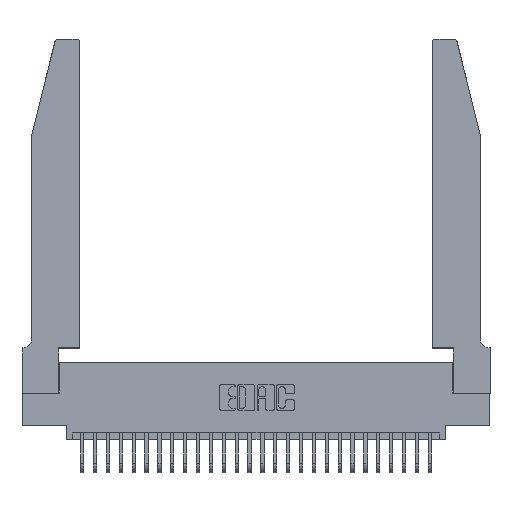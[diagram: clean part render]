
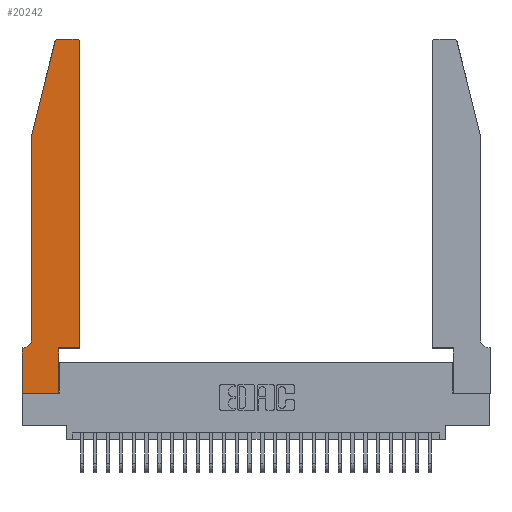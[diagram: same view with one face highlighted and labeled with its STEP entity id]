
A CAD part, top view. The second image highlights one B-rep face of the part: STEP entity #20242.
In plain terms, the highlighted planar face has unit normal (0, 0, 1).
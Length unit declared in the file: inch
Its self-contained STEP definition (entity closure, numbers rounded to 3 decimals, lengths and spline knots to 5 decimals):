
#351 = CARTESIAN_POINT ( 'NONE',  ( 0.2605, 2.75, 0.37 ) ) ;
#544 = DIRECTION ( 'NONE',  ( -1., 0., 0. ) ) ;
#545 = FACE_OUTER_BOUND ( 'NONE', #12466, .T. ) ;
#628 = VECTOR ( 'NONE', #4740, 39.37008 ) ;
#703 = VERTEX_POINT ( 'NONE', #11241 ) ;
#746 = VERTEX_POINT ( 'NONE', #26456 ) ;
#1192 = AXIS2_PLACEMENT_3D ( 'NONE', #9117, #24202, #11315 ) ;
#1303 = CARTESIAN_POINT ( 'NONE',  ( 0.284, 2.75, 0.37 ) ) ;
#1396 = AXIS2_PLACEMENT_3D ( 'NONE', #6137, #21245, #8283 ) ;
#2359 = DIRECTION ( 'NONE',  ( 1., 0., 0. ) ) ;
#2407 = EDGE_CURVE ( 'NONE', #12061, #4541, #15665, .T. ) ;
#2784 = ORIENTED_EDGE ( 'NONE', *, *, #23718, .T. ) ;
#3391 = LINE ( 'NONE', #25448, #25352 ) ;
#3420 = VECTOR ( 'NONE', #4451, 39.37008 ) ;
#3762 = VERTEX_POINT ( 'NONE', #19898 ) ;
#4040 = VERTEX_POINT ( 'NONE', #1303 ) ;
#4061 = CARTESIAN_POINT ( 'NONE',  ( 0.4505, 0.35, 0.37 ) ) ;
#4200 = ORIENTED_EDGE ( 'NONE', *, *, #19794, .T. ) ;
#4275 = CARTESIAN_POINT ( 'NONE',  ( 0.4505, 2.72, 0.37 ) ) ;
#4295 = VERTEX_POINT ( 'NONE', #4275 ) ;
#4451 = DIRECTION ( 'NONE',  ( 0., -1., 0. ) ) ;
#4541 = VERTEX_POINT ( 'NONE', #7356 ) ;
#4579 = CARTESIAN_POINT ( 'NONE',  ( 0., 0., 0.37 ) ) ;
#4740 = DIRECTION ( 'NONE',  ( -1., 0., 0. ) ) ;
#5002 = DIRECTION ( 'NONE',  ( 0., -1., 0. ) ) ;
#5153 = EDGE_CURVE ( 'NONE', #18616, #25102, #11440, .T. ) ;
#5205 = VECTOR ( 'NONE', #8239, 39.37008 ) ;
#5359 = VERTEX_POINT ( 'NONE', #17204 ) ;
#5669 = EDGE_CURVE ( 'NONE', #25165, #4295, #27196, .T. ) ;
#5719 = ORIENTED_EDGE ( 'NONE', *, *, #19094, .T. ) ;
#6094 = CARTESIAN_POINT ( 'NONE',  ( 0.2865, 0.35, 0.37 ) ) ;
#6135 = AXIS2_PLACEMENT_3D ( 'NONE', #13199, #8810, #2359 ) ;
#6137 = CARTESIAN_POINT ( 'NONE',  ( 0.4205, 2.72, 0.37 ) ) ;
#6362 = ORIENTED_EDGE ( 'NONE', *, *, #14368, .T. ) ;
#6398 = CARTESIAN_POINT ( 'NONE',  ( 0.4505, 0.35, 0.37 ) ) ;
#7225 = ORIENTED_EDGE ( 'NONE', *, *, #22177, .T. ) ;
#7356 = CARTESIAN_POINT ( 'NONE',  ( 0., 0., 0.37 ) ) ;
#8239 = DIRECTION ( 'NONE',  ( 0., 1., 0. ) ) ;
#8283 = DIRECTION ( 'NONE',  ( 1., 0., 0. ) ) ;
#8360 = ORIENTED_EDGE ( 'NONE', *, *, #10565, .T. ) ;
#8382 = DIRECTION ( 'NONE',  ( 1., 0., 0. ) ) ;
#8576 = EDGE_CURVE ( 'NONE', #5359, #25165, #22084, .T. ) ;
#8810 = DIRECTION ( 'NONE',  ( 0., 0., 1. ) ) ;
#9089 = ORIENTED_EDGE ( 'NONE', *, *, #25315, .T. ) ;
#9117 = CARTESIAN_POINT ( 'NONE',  ( 0.284, 2.72, 0.37 ) ) ;
#9367 = VECTOR ( 'NONE', #11588, 39.37008 ) ;
#10418 = VECTOR ( 'NONE', #5002, 39.37008 ) ;
#10565 = EDGE_CURVE ( 'NONE', #703, #22980, #3391, .T. ) ;
#11241 = CARTESIAN_POINT ( 'NONE',  ( 0.25487, 2.72718, 0.37 ) ) ;
#11273 = LINE ( 'NONE', #4579, #22072 ) ;
#11315 = DIRECTION ( 'NONE',  ( 1., 0., 0. ) ) ;
#11353 = CARTESIAN_POINT ( 'NONE',  ( 0.0755, 0.35, 0.37 ) ) ;
#11440 = CIRCLE ( 'NONE', #12074, 0.07 ) ;
#11588 = DIRECTION ( 'NONE',  ( 0., 1., 0. ) ) ;
#11896 = DIRECTION ( 'NONE',  ( 0., 0., -1. ) ) ;
#12061 = VERTEX_POINT ( 'NONE', #15784 ) ;
#12074 = AXIS2_PLACEMENT_3D ( 'NONE', #24777, #11896, #26895 ) ;
#12466 = EDGE_LOOP ( 'NONE', ( #5719, #9089, #8360, #4200, #14666, #6362, #24120, #15841, #2784, #18570, #17624, #7225 ) ) ;
#12695 = DIRECTION ( 'NONE',  ( -0.239, -0.971, 0. ) ) ;
#13199 = CARTESIAN_POINT ( 'NONE',  ( 0., 0.35, 0.37 ) ) ;
#13595 = CARTESIAN_POINT ( 'NONE',  ( 0.0755, 0.42, 0.37 ) ) ;
#13609 = CARTESIAN_POINT ( 'NONE',  ( 0.0755, 2., 0.37 ) ) ;
#13804 = CARTESIAN_POINT ( 'NONE',  ( 0.4505, 0.35, 0.37 ) ) ;
#14078 = CIRCLE ( 'NONE', #1396, 0.03 ) ;
#14368 = EDGE_CURVE ( 'NONE', #25102, #12061, #18785, .T. ) ;
#14666 = ORIENTED_EDGE ( 'NONE', *, *, #5153, .T. ) ;
#15277 = CARTESIAN_POINT ( 'NONE',  ( 0., 0., 0.37 ) ) ;
#15407 = PLANE ( 'NONE',  #6135 ) ;
#15665 = LINE ( 'NONE', #15277, #3420 ) ;
#15784 = CARTESIAN_POINT ( 'NONE',  ( 0., 0.35, 0.37 ) ) ;
#15811 = CARTESIAN_POINT ( 'NONE',  ( 0.0755, 2., 0.37 ) ) ;
#15841 = ORIENTED_EDGE ( 'NONE', *, *, #23923, .T. ) ;
#16392 = VECTOR ( 'NONE', #8382, 39.37008 ) ;
#17204 = CARTESIAN_POINT ( 'NONE',  ( 0.2865, 0.35, 0.37 ) ) ;
#17462 = VECTOR ( 'NONE', #544, 39.37008 ) ;
#17624 = ORIENTED_EDGE ( 'NONE', *, *, #5669, .T. ) ;
#17648 = DIRECTION ( 'NONE',  ( 1., 0., 0. ) ) ;
#18570 = ORIENTED_EDGE ( 'NONE', *, *, #8576, .T. ) ;
#18616 = VERTEX_POINT ( 'NONE', #13595 ) ;
#18785 = LINE ( 'NONE', #11353, #17462 ) ;
#19094 = EDGE_CURVE ( 'NONE', #3762, #4040, #22281, .T. ) ;
#19794 = EDGE_CURVE ( 'NONE', #22980, #18616, #23223, .T. ) ;
#19898 = CARTESIAN_POINT ( 'NONE',  ( 0.4205, 2.75, 0.37 ) ) ;
#20242 = ADVANCED_FACE ( 'NONE', ( #545 ), #15407, .T. ) ;
#21245 = DIRECTION ( 'NONE',  ( 0., 0., 1. ) ) ;
#22072 = VECTOR ( 'NONE', #17648, 39.37008 ) ;
#22084 = LINE ( 'NONE', #4061, #16392 ) ;
#22177 = EDGE_CURVE ( 'NONE', #4295, #3762, #14078, .T. ) ;
#22281 = LINE ( 'NONE', #351, #628 ) ;
#22417 = LINE ( 'NONE', #6094, #5205 ) ;
#22980 = VERTEX_POINT ( 'NONE', #13609 ) ;
#23223 = LINE ( 'NONE', #15811, #10418 ) ;
#23718 = EDGE_CURVE ( 'NONE', #746, #5359, #22417, .T. ) ;
#23923 = EDGE_CURVE ( 'NONE', #4541, #746, #11273, .T. ) ;
#24120 = ORIENTED_EDGE ( 'NONE', *, *, #2407, .T. ) ;
#24202 = DIRECTION ( 'NONE',  ( 0., 0., 1. ) ) ;
#24777 = CARTESIAN_POINT ( 'NONE',  ( 0.0055, 0.42, 0.37 ) ) ;
#25102 = VERTEX_POINT ( 'NONE', #27657 ) ;
#25165 = VERTEX_POINT ( 'NONE', #6398 ) ;
#25315 = EDGE_CURVE ( 'NONE', #4040, #703, #26989, .T. ) ;
#25352 = VECTOR ( 'NONE', #12695, 39.37008 ) ;
#25448 = CARTESIAN_POINT ( 'NONE',  ( 0.0755, 2., 0.37 ) ) ;
#26456 = CARTESIAN_POINT ( 'NONE',  ( 0.2865, 0., 0.37 ) ) ;
#26895 = DIRECTION ( 'NONE',  ( -1., 0., 0. ) ) ;
#26989 = CIRCLE ( 'NONE', #1192, 0.03 ) ;
#27196 = LINE ( 'NONE', #13804, #9367 ) ;
#27657 = CARTESIAN_POINT ( 'NONE',  ( 0.0055, 0.35, 0.37 ) ) ;
